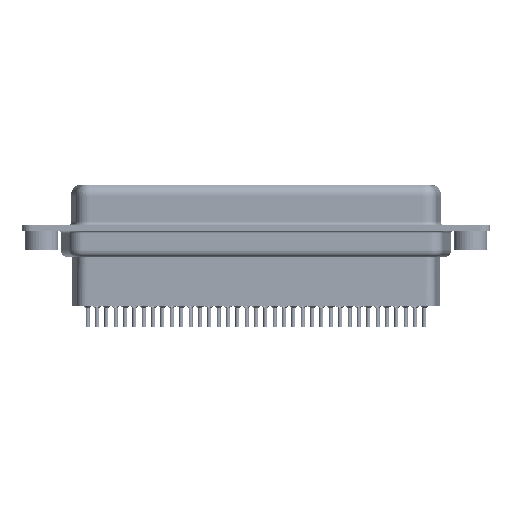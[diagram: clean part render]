
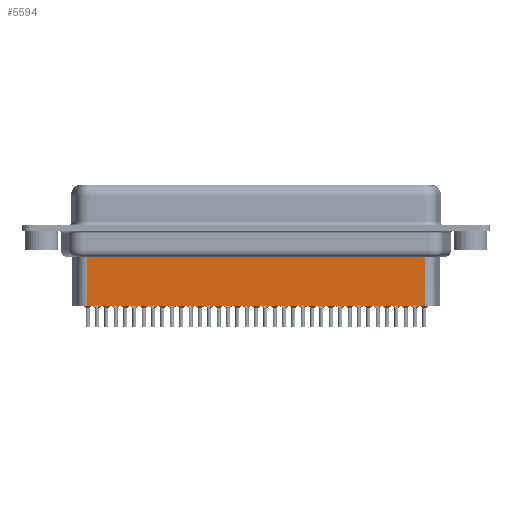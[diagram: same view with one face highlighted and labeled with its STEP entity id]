
A CAD part, front view. The second image highlights one B-rep face of the part: STEP entity #5594.
In plain terms, the highlighted planar face has unit normal (0, -1, 0).
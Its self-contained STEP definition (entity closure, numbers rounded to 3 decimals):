
#1697 = VECTOR ( 'NONE', #15943, 1000. ) ;
#5235 = ORIENTED_EDGE ( 'NONE', *, *, #17359, .T. ) ;
#5300 = VERTEX_POINT ( 'NONE', #23643 ) ;
#5594 = ADVANCED_FACE ( 'NONE', ( #28257 ), #27279, .T. ) ;
#6487 = VERTEX_POINT ( 'NONE', #6714 ) ;
#6494 = VERTEX_POINT ( 'NONE', #6822 ) ;
#6601 = EDGE_LOOP ( 'NONE', ( #10250, #5235, #15286, #7549 ) ) ;
#6714 = CARTESIAN_POINT ( 'NONE',  ( 6.706, -3.5, -4.097 ) ) ;
#6822 = CARTESIAN_POINT ( 'NONE',  ( 6.706, -3.5, -11.45 ) ) ;
#7549 = ORIENTED_EDGE ( 'NONE', *, *, #25001, .F. ) ;
#7778 = DIRECTION ( 'NONE',  ( 0., 0., -1. ) ) ;
#8280 = LINE ( 'NONE', #25750, #1697 ) ;
#9598 = LINE ( 'NONE', #21769, #27630 ) ;
#9805 = LINE ( 'NONE', #25074, #21357 ) ;
#10250 = ORIENTED_EDGE ( 'NONE', *, *, #23216, .F. ) ;
#10458 = DIRECTION ( 'NONE',  ( -1., 0., 0. ) ) ;
#12781 = CARTESIAN_POINT ( 'NONE',  ( 56.794, -3.5, -3.1 ) ) ;
#15107 = DIRECTION ( 'NONE',  ( 1., 0., 0. ) ) ;
#15286 = ORIENTED_EDGE ( 'NONE', *, *, #21746, .T. ) ;
#15943 = DIRECTION ( 'NONE',  ( -1., 0., 0. ) ) ;
#16470 = VECTOR ( 'NONE', #7778, 1000. ) ;
#17239 = VERTEX_POINT ( 'NONE', #28462 ) ;
#17267 = AXIS2_PLACEMENT_3D ( 'NONE', #19970, #29757, #15107 ) ;
#17359 = EDGE_CURVE ( 'NONE', #17239, #6487, #9805, .T. ) ;
#18834 = LINE ( 'NONE', #12781, #16470 ) ;
#19970 = CARTESIAN_POINT ( 'NONE',  ( 6.706, -3.5, -3.1 ) ) ;
#21357 = VECTOR ( 'NONE', #10458, 1000. ) ;
#21746 = EDGE_CURVE ( 'NONE', #6487, #6494, #9598, .T. ) ;
#21769 = CARTESIAN_POINT ( 'NONE',  ( 6.706, -3.5, -3.1 ) ) ;
#23216 = EDGE_CURVE ( 'NONE', #17239, #5300, #18834, .T. ) ;
#23643 = CARTESIAN_POINT ( 'NONE',  ( 56.794, -3.5, -11.45 ) ) ;
#25001 = EDGE_CURVE ( 'NONE', #5300, #6494, #8280, .T. ) ;
#25074 = CARTESIAN_POINT ( 'NONE',  ( 6.459, -3.5, -4.097 ) ) ;
#25750 = CARTESIAN_POINT ( 'NONE',  ( 6.706, -3.5, -11.45 ) ) ;
#26653 = DIRECTION ( 'NONE',  ( 0., 0., -1. ) ) ;
#27279 = PLANE ( 'NONE',  #17267 ) ;
#27630 = VECTOR ( 'NONE', #26653, 1000. ) ;
#28257 = FACE_OUTER_BOUND ( 'NONE', #6601, .T. ) ;
#28462 = CARTESIAN_POINT ( 'NONE',  ( 56.794, -3.5, -4.097 ) ) ;
#29757 = DIRECTION ( 'NONE',  ( 0., -1., 0. ) ) ;
